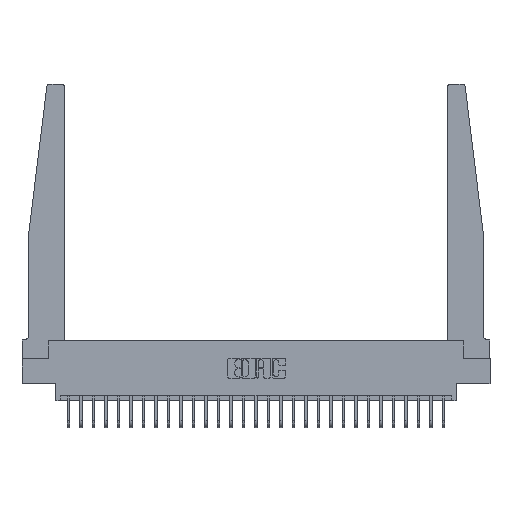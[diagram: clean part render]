
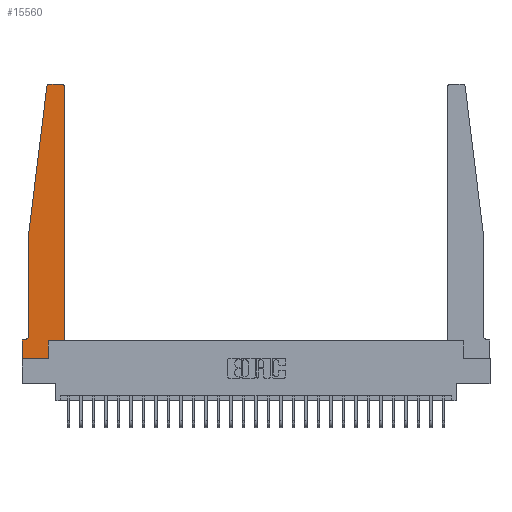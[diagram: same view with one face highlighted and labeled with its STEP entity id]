
A CAD part, top view. The second image highlights one B-rep face of the part: STEP entity #15560.
In plain terms, the highlighted planar face has unit normal (0, 0, 1).
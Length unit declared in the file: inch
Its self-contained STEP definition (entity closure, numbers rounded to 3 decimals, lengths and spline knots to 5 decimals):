
#18 = CARTESIAN_POINT ( 'NONE',  ( 0.425, 0.18, 0.37 ) ) ;
#102 = DIRECTION ( 'NONE',  ( 1., 0., 0. ) ) ;
#166 = ORIENTED_EDGE ( 'NONE', *, *, #16406, .T. ) ;
#470 = VERTEX_POINT ( 'NONE', #17019 ) ;
#651 = DIRECTION ( 'NONE',  ( 0., 0., 1. ) ) ;
#1020 = DIRECTION ( 'NONE',  ( -1., 0., 0. ) ) ;
#1100 = ORIENTED_EDGE ( 'NONE', *, *, #13260, .T. ) ;
#1234 = CARTESIAN_POINT ( 'NONE',  ( 0.425, 0.18, 0.37 ) ) ;
#2070 = LINE ( 'NONE', #10251, #16420 ) ;
#2287 = DIRECTION ( 'NONE',  ( 0., 0., -1. ) ) ;
#2591 = CIRCLE ( 'NONE', #18185, 0.03 ) ;
#2751 = EDGE_LOOP ( 'NONE', ( #12411, #5598, #16581, #9667, #3414, #166, #21992, #16098, #4700, #16164, #1100, #6794 ) ) ;
#2994 = LINE ( 'NONE', #12510, #25781 ) ;
#3338 = LINE ( 'NONE', #1234, #5928 ) ;
#3414 = ORIENTED_EDGE ( 'NONE', *, *, #3469, .T. ) ;
#3469 = EDGE_CURVE ( 'NONE', #10900, #25957, #24563, .T. ) ;
#3874 = VECTOR ( 'NONE', #7779, 39.37008 ) ;
#4080 = EDGE_CURVE ( 'NONE', #4887, #8264, #18074, .T. ) ;
#4374 = CARTESIAN_POINT ( 'NONE',  ( 0.27653, 2.75, 0.37 ) ) ;
#4677 = DIRECTION ( 'NONE',  ( -1., 0., 0. ) ) ;
#4700 = ORIENTED_EDGE ( 'NONE', *, *, #15222, .T. ) ;
#4887 = VERTEX_POINT ( 'NONE', #7303 ) ;
#5468 = CARTESIAN_POINT ( 'NONE',  ( 0.065, 1.25, 0.37 ) ) ;
#5551 = CARTESIAN_POINT ( 'NONE',  ( 0.065, 1.25, 0.37 ) ) ;
#5598 = ORIENTED_EDGE ( 'NONE', *, *, #15874, .T. ) ;
#5928 = VECTOR ( 'NONE', #23451, 39.37008 ) ;
#6601 = CARTESIAN_POINT ( 'NONE',  ( 0.27653, 2.72, 0.37 ) ) ;
#6779 = VECTOR ( 'NONE', #11942, 39.37008 ) ;
#6794 = ORIENTED_EDGE ( 'NONE', *, *, #7434, .T. ) ;
#7303 = CARTESIAN_POINT ( 'NONE',  ( 0., 0.1875, 0.37 ) ) ;
#7434 = EDGE_CURVE ( 'NONE', #470, #13740, #12800, .T. ) ;
#7779 = DIRECTION ( 'NONE',  ( 0., -1., 0. ) ) ;
#8264 = VERTEX_POINT ( 'NONE', #16248 ) ;
#8474 = VERTEX_POINT ( 'NONE', #9401 ) ;
#8742 = VERTEX_POINT ( 'NONE', #18360 ) ;
#8945 = DIRECTION ( 'NONE',  ( 0., 0., 1. ) ) ;
#9065 = DIRECTION ( 'NONE',  ( -1., 0., 0. ) ) ;
#9401 = CARTESIAN_POINT ( 'NONE',  ( 0.065, 1.25, 0.37 ) ) ;
#9515 = DIRECTION ( 'NONE',  ( 0., 0., 1. ) ) ;
#9582 = CARTESIAN_POINT ( 'NONE',  ( 0.065, 0.1875, 0.37 ) ) ;
#9667 = ORIENTED_EDGE ( 'NONE', *, *, #22657, .T. ) ;
#10251 = CARTESIAN_POINT ( 'NONE',  ( 0., 0., 0.37 ) ) ;
#10335 = VERTEX_POINT ( 'NONE', #25892 ) ;
#10476 = CARTESIAN_POINT ( 'NONE',  ( 0.2605, 0., 0.37 ) ) ;
#10745 = VERTEX_POINT ( 'NONE', #4374 ) ;
#10900 = VERTEX_POINT ( 'NONE', #18759 ) ;
#11289 = EDGE_CURVE ( 'NONE', #13740, #10745, #2994, .T. ) ;
#11522 = LINE ( 'NONE', #5468, #19883 ) ;
#11729 = LINE ( 'NONE', #5551, #18801 ) ;
#11905 = CARTESIAN_POINT ( 'NONE',  ( 0.2605, 0.18, 0.37 ) ) ;
#11942 = DIRECTION ( 'NONE',  ( 0., 1., 0. ) ) ;
#12079 = VERTEX_POINT ( 'NONE', #10476 ) ;
#12411 = ORIENTED_EDGE ( 'NONE', *, *, #11289, .T. ) ;
#12510 = CARTESIAN_POINT ( 'NONE',  ( 0.25, 2.75, 0.37 ) ) ;
#12800 = CIRCLE ( 'NONE', #15343, 0.03 ) ;
#12822 = EDGE_CURVE ( 'NONE', #8264, #12079, #2070, .T. ) ;
#13083 = VERTEX_POINT ( 'NONE', #18 ) ;
#13097 = CARTESIAN_POINT ( 'NONE',  ( 0.015, 0.1875, 0.37 ) ) ;
#13260 = EDGE_CURVE ( 'NONE', #13083, #470, #13777, .T. ) ;
#13450 = EDGE_CURVE ( 'NONE', #8742, #13083, #3338, .T. ) ;
#13740 = VERTEX_POINT ( 'NONE', #19688 ) ;
#13777 = LINE ( 'NONE', #23886, #6779 ) ;
#13879 = LINE ( 'NONE', #11905, #18601 ) ;
#14367 = AXIS2_PLACEMENT_3D ( 'NONE', #23822, #9515, #19300 ) ;
#14674 = CARTESIAN_POINT ( 'NONE',  ( 0.015, 0.2375, 0.37 ) ) ;
#14983 = LINE ( 'NONE', #9582, #17380 ) ;
#14987 = CARTESIAN_POINT ( 'NONE',  ( 0.395, 2.72, 0.37 ) ) ;
#15086 = EDGE_CURVE ( 'NONE', #10335, #8474, #11522, .T. ) ;
#15222 = EDGE_CURVE ( 'NONE', #12079, #8742, #13879, .T. ) ;
#15343 = AXIS2_PLACEMENT_3D ( 'NONE', #14987, #8945, #22581 ) ;
#15560 = ADVANCED_FACE ( 'NONE', ( #17443 ), #21961, .T. ) ;
#15874 = EDGE_CURVE ( 'NONE', #10745, #10335, #2591, .T. ) ;
#16098 = ORIENTED_EDGE ( 'NONE', *, *, #12822, .T. ) ;
#16164 = ORIENTED_EDGE ( 'NONE', *, *, #13450, .T. ) ;
#16248 = CARTESIAN_POINT ( 'NONE',  ( 0., 0., 0.37 ) ) ;
#16406 = EDGE_CURVE ( 'NONE', #25957, #4887, #14983, .T. ) ;
#16420 = VECTOR ( 'NONE', #102, 39.37008 ) ;
#16581 = ORIENTED_EDGE ( 'NONE', *, *, #15086, .T. ) ;
#16878 = DIRECTION ( 'NONE',  ( 1., 0., 0. ) ) ;
#17019 = CARTESIAN_POINT ( 'NONE',  ( 0.425, 2.72, 0.37 ) ) ;
#17380 = VECTOR ( 'NONE', #9065, 39.37008 ) ;
#17443 = FACE_OUTER_BOUND ( 'NONE', #2751, .T. ) ;
#17815 = CARTESIAN_POINT ( 'NONE',  ( 0., 0., 0.37 ) ) ;
#18074 = LINE ( 'NONE', #17815, #3874 ) ;
#18185 = AXIS2_PLACEMENT_3D ( 'NONE', #6601, #651, #16878 ) ;
#18360 = CARTESIAN_POINT ( 'NONE',  ( 0.2605, 0.18, 0.37 ) ) ;
#18601 = VECTOR ( 'NONE', #19996, 39.37008 ) ;
#18759 = CARTESIAN_POINT ( 'NONE',  ( 0.065, 0.2375, 0.37 ) ) ;
#18801 = VECTOR ( 'NONE', #22195, 39.37008 ) ;
#19300 = DIRECTION ( 'NONE',  ( 1., 0., 0. ) ) ;
#19611 = DIRECTION ( 'NONE',  ( -0.122, -0.992, 0. ) ) ;
#19688 = CARTESIAN_POINT ( 'NONE',  ( 0.395, 2.75, 0.37 ) ) ;
#19883 = VECTOR ( 'NONE', #19611, 39.37008 ) ;
#19996 = DIRECTION ( 'NONE',  ( 0., 1., 0. ) ) ;
#21961 = PLANE ( 'NONE',  #14367 ) ;
#21992 = ORIENTED_EDGE ( 'NONE', *, *, #4080, .T. ) ;
#22195 = DIRECTION ( 'NONE',  ( 0., -1., 0. ) ) ;
#22581 = DIRECTION ( 'NONE',  ( 1., 0., 0. ) ) ;
#22657 = EDGE_CURVE ( 'NONE', #8474, #10900, #11729, .T. ) ;
#23268 = AXIS2_PLACEMENT_3D ( 'NONE', #14674, #2287, #4677 ) ;
#23451 = DIRECTION ( 'NONE',  ( 1., 0., 0. ) ) ;
#23822 = CARTESIAN_POINT ( 'NONE',  ( 0., 0.1875, 0.37 ) ) ;
#23886 = CARTESIAN_POINT ( 'NONE',  ( 0.425, 0.18, 0.37 ) ) ;
#24563 = CIRCLE ( 'NONE', #23268, 0.05 ) ;
#25781 = VECTOR ( 'NONE', #1020, 39.37008 ) ;
#25892 = CARTESIAN_POINT ( 'NONE',  ( 0.24675, 2.72367, 0.37 ) ) ;
#25957 = VERTEX_POINT ( 'NONE', #13097 ) ;
